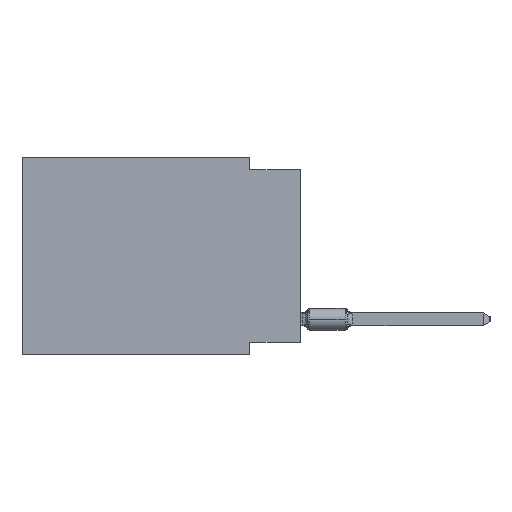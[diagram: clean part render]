
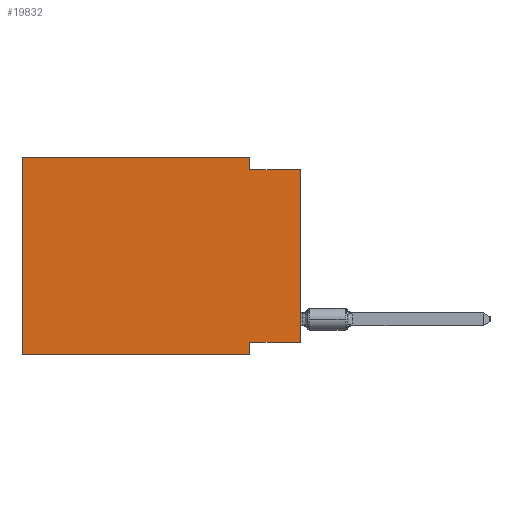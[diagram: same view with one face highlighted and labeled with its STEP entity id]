
A CAD part, left-side view. The second image highlights one B-rep face of the part: STEP entity #19832.
In plain terms, the highlighted planar face has unit normal (-1, 0, 0).
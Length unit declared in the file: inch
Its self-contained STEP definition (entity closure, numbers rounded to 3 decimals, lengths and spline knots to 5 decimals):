
#970 = DIRECTION ( 'NONE',  ( 0., 1., 0. ) ) ;
#1108 = ORIENTED_EDGE ( 'NONE', *, *, #6978, .T. ) ;
#1361 = DIRECTION ( 'NONE',  ( 0., 0., -1. ) ) ;
#1419 = LINE ( 'NONE', #13066, #6599 ) ;
#2357 = ORIENTED_EDGE ( 'NONE', *, *, #12866, .F. ) ;
#2586 = CARTESIAN_POINT ( 'NONE',  ( 0., 0.55, -0.39 ) ) ;
#3197 = CARTESIAN_POINT ( 'NONE',  ( 0., 0., -0.025 ) ) ;
#4306 = VERTEX_POINT ( 'NONE', #7111 ) ;
#4426 = VERTEX_POINT ( 'NONE', #21793 ) ;
#4836 = LINE ( 'NONE', #8198, #5994 ) ;
#4857 = CARTESIAN_POINT ( 'NONE',  ( 0., 0., 0. ) ) ;
#5089 = DIRECTION ( 'NONE',  ( 0., -1., 0. ) ) ;
#5163 = VECTOR ( 'NONE', #21428, 39.37008 ) ;
#5994 = VECTOR ( 'NONE', #15330, 39.37008 ) ;
#6232 = EDGE_CURVE ( 'NONE', #28136, #29397, #14013, .T. ) ;
#6497 = FACE_OUTER_BOUND ( 'NONE', #26166, .T. ) ;
#6599 = VECTOR ( 'NONE', #970, 39.37008 ) ;
#6978 = EDGE_CURVE ( 'NONE', #23614, #4306, #30296, .T. ) ;
#7111 = CARTESIAN_POINT ( 'NONE',  ( 0., 0.1, -0.39 ) ) ;
#7858 = VERTEX_POINT ( 'NONE', #25428 ) ;
#8006 = DIRECTION ( 'NONE',  ( 0., -1., 0. ) ) ;
#8198 = CARTESIAN_POINT ( 'NONE',  ( 0., 0.1, 0. ) ) ;
#9032 = CARTESIAN_POINT ( 'NONE',  ( 0., 0., -0.025 ) ) ;
#10164 = ORIENTED_EDGE ( 'NONE', *, *, #18758, .F. ) ;
#10297 = EDGE_CURVE ( 'NONE', #13164, #4306, #21946, .T. ) ;
#10346 = CARTESIAN_POINT ( 'NONE',  ( 0., 0.1, -0.39 ) ) ;
#10872 = VECTOR ( 'NONE', #5089, 39.37008 ) ;
#10891 = VECTOR ( 'NONE', #19622, 39.37008 ) ;
#10922 = AXIS2_PLACEMENT_3D ( 'NONE', #13160, #29856, #1361 ) ;
#12671 = ORIENTED_EDGE ( 'NONE', *, *, #10297, .F. ) ;
#12866 = EDGE_CURVE ( 'NONE', #4426, #29397, #14986, .T. ) ;
#13066 = CARTESIAN_POINT ( 'NONE',  ( 0., 0., -0.365 ) ) ;
#13160 = CARTESIAN_POINT ( 'NONE',  ( 0., 0.55, 0. ) ) ;
#13164 = VERTEX_POINT ( 'NONE', #26062 ) ;
#14013 = LINE ( 'NONE', #4857, #30434 ) ;
#14059 = DIRECTION ( 'NONE',  ( 0., -1., 0. ) ) ;
#14170 = ORIENTED_EDGE ( 'NONE', *, *, #6232, .T. ) ;
#14312 = DIRECTION ( 'NONE',  ( 0., 0., 1. ) ) ;
#14986 = LINE ( 'NONE', #3197, #20799 ) ;
#15330 = DIRECTION ( 'NONE',  ( 0., 0., -1. ) ) ;
#16406 = LINE ( 'NONE', #23489, #10872 ) ;
#18254 = PLANE ( 'NONE',  #10922 ) ;
#18445 = EDGE_CURVE ( 'NONE', #7858, #4426, #4836, .T. ) ;
#18469 = ORIENTED_EDGE ( 'NONE', *, *, #29252, .F. ) ;
#18758 = EDGE_CURVE ( 'NONE', #28936, #7858, #16406, .T. ) ;
#18769 = CARTESIAN_POINT ( 'NONE',  ( 0., 0.55, -0.39 ) ) ;
#19622 = DIRECTION ( 'NONE',  ( 0., 0., -1. ) ) ;
#19832 = ADVANCED_FACE ( 'NONE', ( #6497 ), #18254, .F. ) ;
#20799 = VECTOR ( 'NONE', #8006, 39.37008 ) ;
#20817 = LINE ( 'NONE', #30258, #5163 ) ;
#21428 = DIRECTION ( 'NONE',  ( 0., 0., 1. ) ) ;
#21793 = CARTESIAN_POINT ( 'NONE',  ( 0., 0.1, -0.025 ) ) ;
#21946 = LINE ( 'NONE', #10346, #10891 ) ;
#22798 = VECTOR ( 'NONE', #14059, 39.37008 ) ;
#22901 = CARTESIAN_POINT ( 'NONE',  ( 0., 0., -0.365 ) ) ;
#23489 = CARTESIAN_POINT ( 'NONE',  ( 0., 0.55, 0. ) ) ;
#23614 = VERTEX_POINT ( 'NONE', #18769 ) ;
#25428 = CARTESIAN_POINT ( 'NONE',  ( 0., 0.1, 0. ) ) ;
#25541 = ORIENTED_EDGE ( 'NONE', *, *, #18445, .F. ) ;
#26062 = CARTESIAN_POINT ( 'NONE',  ( 0., 0.1, -0.365 ) ) ;
#26166 = EDGE_LOOP ( 'NONE', ( #14170, #2357, #25541, #10164, #27758, #1108, #12671, #18469 ) ) ;
#27758 = ORIENTED_EDGE ( 'NONE', *, *, #30284, .F. ) ;
#28136 = VERTEX_POINT ( 'NONE', #22901 ) ;
#28936 = VERTEX_POINT ( 'NONE', #29478 ) ;
#29252 = EDGE_CURVE ( 'NONE', #28136, #13164, #1419, .T. ) ;
#29397 = VERTEX_POINT ( 'NONE', #9032 ) ;
#29478 = CARTESIAN_POINT ( 'NONE',  ( 0., 0.55, 0. ) ) ;
#29856 = DIRECTION ( 'NONE',  ( 1., 0., 0. ) ) ;
#30258 = CARTESIAN_POINT ( 'NONE',  ( 0., 0.55, 0. ) ) ;
#30284 = EDGE_CURVE ( 'NONE', #23614, #28936, #20817, .T. ) ;
#30296 = LINE ( 'NONE', #2586, #22798 ) ;
#30434 = VECTOR ( 'NONE', #14312, 39.37008 ) ;
